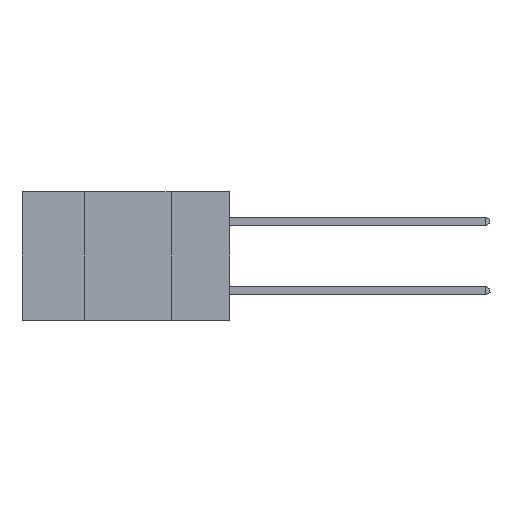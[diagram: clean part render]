
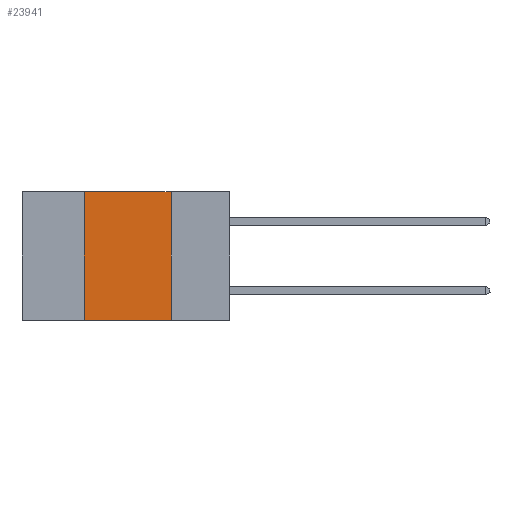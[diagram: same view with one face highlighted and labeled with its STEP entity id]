
A CAD part, left-side view. The second image highlights one B-rep face of the part: STEP entity #23941.
In plain terms, the highlighted planar face has unit normal (-1, 0, 0).
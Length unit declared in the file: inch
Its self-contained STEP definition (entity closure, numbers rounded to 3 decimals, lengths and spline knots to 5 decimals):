
#740 = EDGE_CURVE ( 'NONE', #5256, #29903, #3997, .T. ) ;
#873 = LINE ( 'NONE', #4044, #6565 ) ;
#1039 = PLANE ( 'NONE',  #14994 ) ;
#1624 = VERTEX_POINT ( 'NONE', #23523 ) ;
#1705 = DIRECTION ( 'NONE',  ( 0., 0., -1. ) ) ;
#1763 = ORIENTED_EDGE ( 'NONE', *, *, #740, .T. ) ;
#2044 = EDGE_LOOP ( 'NONE', ( #9148, #5677, #3916, #1763 ) ) ;
#3425 = DIRECTION ( 'NONE',  ( 0., -1., 0. ) ) ;
#3708 = DIRECTION ( 'NONE',  ( 0., 0., -1. ) ) ;
#3916 = ORIENTED_EDGE ( 'NONE', *, *, #15985, .F. ) ;
#3997 = LINE ( 'NONE', #27705, #12714 ) ;
#4044 = CARTESIAN_POINT ( 'NONE',  ( 0., 0.17, 0. ) ) ;
#4533 = FACE_OUTER_BOUND ( 'NONE', #2044, .T. ) ;
#5256 = VERTEX_POINT ( 'NONE', #31073 ) ;
#5677 = ORIENTED_EDGE ( 'NONE', *, *, #8089, .F. ) ;
#6565 = VECTOR ( 'NONE', #1705, 39.37008 ) ;
#8089 = EDGE_CURVE ( 'NONE', #17580, #1624, #19375, .T. ) ;
#9096 = CARTESIAN_POINT ( 'NONE',  ( 0., 0.42, 0. ) ) ;
#9148 = ORIENTED_EDGE ( 'NONE', *, *, #13998, .F. ) ;
#9854 = VECTOR ( 'NONE', #27547, 39.37008 ) ;
#10560 = CARTESIAN_POINT ( 'NONE',  ( 0., 0.6, 0. ) ) ;
#10561 = DIRECTION ( 'NONE',  ( 0., 0., 1. ) ) ;
#12714 = VECTOR ( 'NONE', #3425, 39.37008 ) ;
#13991 = CARTESIAN_POINT ( 'NONE',  ( 0., 0.17, -0.37 ) ) ;
#13998 = EDGE_CURVE ( 'NONE', #1624, #29903, #873, .T. ) ;
#14994 = AXIS2_PLACEMENT_3D ( 'NONE', #27774, #27987, #3708 ) ;
#15985 = EDGE_CURVE ( 'NONE', #5256, #17580, #25573, .T. ) ;
#16108 = VECTOR ( 'NONE', #10561, 39.37008 ) ;
#17580 = VERTEX_POINT ( 'NONE', #9096 ) ;
#19375 = LINE ( 'NONE', #10560, #9854 ) ;
#22897 = CARTESIAN_POINT ( 'NONE',  ( 0., 0.42, 0. ) ) ;
#23523 = CARTESIAN_POINT ( 'NONE',  ( 0., 0.17, 0. ) ) ;
#23941 = ADVANCED_FACE ( 'NONE', ( #4533 ), #1039, .F. ) ;
#25573 = LINE ( 'NONE', #22897, #16108 ) ;
#27547 = DIRECTION ( 'NONE',  ( 0., -1., 0. ) ) ;
#27705 = CARTESIAN_POINT ( 'NONE',  ( 0., 0.6, -0.37 ) ) ;
#27774 = CARTESIAN_POINT ( 'NONE',  ( 0., 0.6, 0. ) ) ;
#27987 = DIRECTION ( 'NONE',  ( 1., 0., 0. ) ) ;
#29903 = VERTEX_POINT ( 'NONE', #13991 ) ;
#31073 = CARTESIAN_POINT ( 'NONE',  ( 0., 0.42, -0.37 ) ) ;
